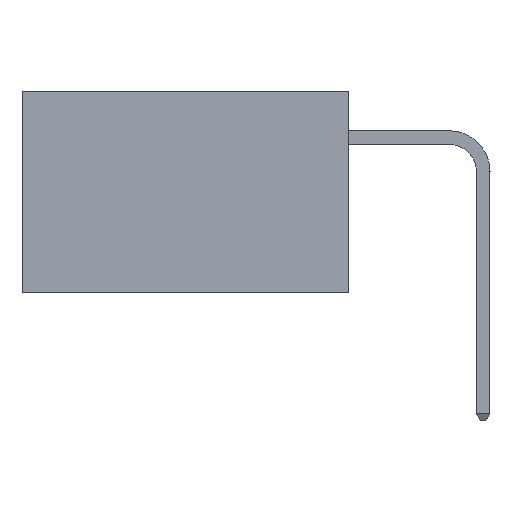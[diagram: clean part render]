
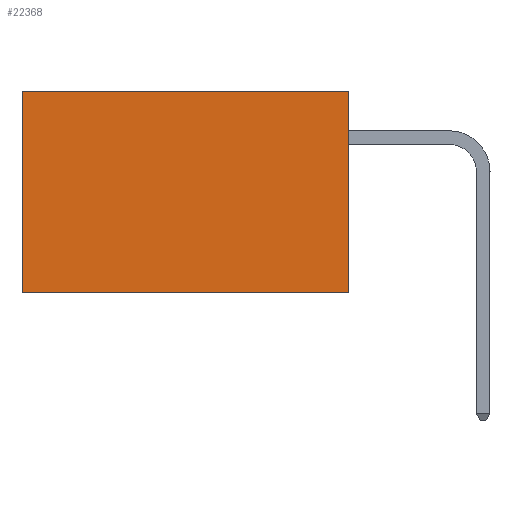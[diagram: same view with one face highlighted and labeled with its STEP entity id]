
A CAD part, left-side view. The second image highlights one B-rep face of the part: STEP entity #22368.
In plain terms, the highlighted planar face has unit normal (-1, 0, 0).
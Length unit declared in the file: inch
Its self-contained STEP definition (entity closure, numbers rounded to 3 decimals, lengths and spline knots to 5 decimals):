
#512 = DIRECTION ( 'NONE',  ( 1., 0., 0. ) ) ;
#1557 = DIRECTION ( 'NONE',  ( 0., 0., -1. ) ) ;
#1876 = CARTESIAN_POINT ( 'NONE',  ( 0.2875, 0., -0.37 ) ) ;
#2223 = VECTOR ( 'NONE', #34377, 39.37008 ) ;
#3665 = EDGE_CURVE ( 'NONE', #33200, #26910, #37726, .T. ) ;
#4573 = DIRECTION ( 'NONE',  ( 0., 1., 0. ) ) ;
#4575 = ORIENTED_EDGE ( 'NONE', *, *, #21366, .F. ) ;
#7607 = EDGE_CURVE ( 'NONE', #12901, #16359, #17040, .T. ) ;
#8912 = CARTESIAN_POINT ( 'NONE',  ( 0.2875, 0.6, -0.37 ) ) ;
#9282 = VECTOR ( 'NONE', #1557, 39.37008 ) ;
#12774 = LINE ( 'NONE', #19674, #2223 ) ;
#12901 = VERTEX_POINT ( 'NONE', #35892 ) ;
#13940 = LINE ( 'NONE', #19144, #20837 ) ;
#14755 = EDGE_CURVE ( 'NONE', #33200, #12901, #13940, .T. ) ;
#15218 = VECTOR ( 'NONE', #34042, 39.37008 ) ;
#16147 = EDGE_LOOP ( 'NONE', ( #28298, #4575, #30388, #32847 ) ) ;
#16359 = VERTEX_POINT ( 'NONE', #8912 ) ;
#17040 = LINE ( 'NONE', #18992, #9282 ) ;
#18129 = PLANE ( 'NONE',  #32489 ) ;
#18722 = CARTESIAN_POINT ( 'NONE',  ( 0.2875, 0., 0. ) ) ;
#18992 = CARTESIAN_POINT ( 'NONE',  ( 0.2875, 0.6, 0. ) ) ;
#19144 = CARTESIAN_POINT ( 'NONE',  ( 0.2875, 0., 0. ) ) ;
#19674 = CARTESIAN_POINT ( 'NONE',  ( 0.2875, 0., -0.37 ) ) ;
#20837 = VECTOR ( 'NONE', #4573, 39.37008 ) ;
#21065 = DIRECTION ( 'NONE',  ( 0., 0., -1. ) ) ;
#21366 = EDGE_CURVE ( 'NONE', #26910, #16359, #12774, .T. ) ;
#22368 = ADVANCED_FACE ( 'NONE', ( #38008 ), #18129, .F. ) ;
#23946 = CARTESIAN_POINT ( 'NONE',  ( 0.2875, 0., 0. ) ) ;
#26910 = VERTEX_POINT ( 'NONE', #1876 ) ;
#28298 = ORIENTED_EDGE ( 'NONE', *, *, #7607, .T. ) ;
#30388 = ORIENTED_EDGE ( 'NONE', *, *, #3665, .F. ) ;
#32489 = AXIS2_PLACEMENT_3D ( 'NONE', #23946, #512, #21065 ) ;
#32847 = ORIENTED_EDGE ( 'NONE', *, *, #14755, .T. ) ;
#33200 = VERTEX_POINT ( 'NONE', #18722 ) ;
#34042 = DIRECTION ( 'NONE',  ( 0., 0., -1. ) ) ;
#34377 = DIRECTION ( 'NONE',  ( 0., 1., 0. ) ) ;
#35892 = CARTESIAN_POINT ( 'NONE',  ( 0.2875, 0.6, 0. ) ) ;
#36752 = CARTESIAN_POINT ( 'NONE',  ( 0.2875, 0., 0. ) ) ;
#37726 = LINE ( 'NONE', #36752, #15218 ) ;
#38008 = FACE_OUTER_BOUND ( 'NONE', #16147, .T. ) ;
